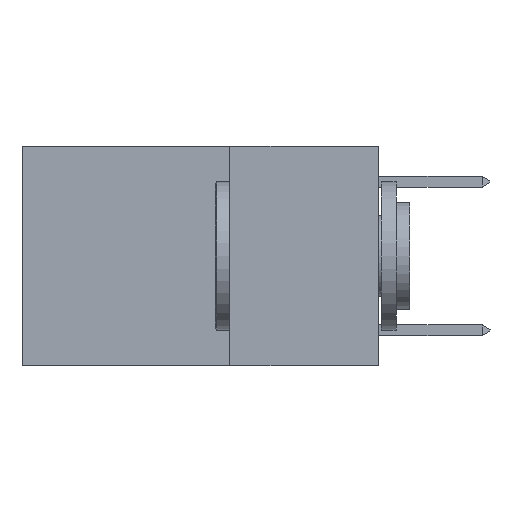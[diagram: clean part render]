
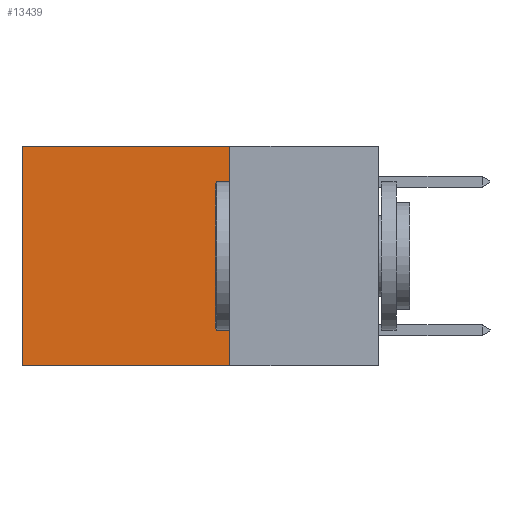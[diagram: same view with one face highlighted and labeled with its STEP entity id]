
A CAD part, left-side view. The second image highlights one B-rep face of the part: STEP entity #13439.
In plain terms, the highlighted planar face has unit normal (-1, 0, 0).
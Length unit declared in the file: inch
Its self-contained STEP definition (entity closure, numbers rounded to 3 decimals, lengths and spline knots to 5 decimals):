
#74 = AXIS2_PLACEMENT_3D ( 'NONE', #9755, #10121, #9610 ) ;
#887 = CARTESIAN_POINT ( 'NONE',  ( 0.2625, 0.25, -0.37 ) ) ;
#1999 = VERTEX_POINT ( 'NONE', #17537 ) ;
#2059 = DIRECTION ( 'NONE',  ( 0., 1., 0. ) ) ;
#2319 = CARTESIAN_POINT ( 'NONE',  ( 0.2625, 0.25, -0.37 ) ) ;
#3209 = DIRECTION ( 'NONE',  ( 0., 0., -1. ) ) ;
#3644 = CARTESIAN_POINT ( 'NONE',  ( 0.2625, 0.25, 0. ) ) ;
#4474 = ORIENTED_EDGE ( 'NONE', *, *, #15202, .T. ) ;
#4477 = EDGE_LOOP ( 'NONE', ( #7351, #19749, #8187, #4474 ) ) ;
#4479 = DIRECTION ( 'NONE',  ( 0., 1., 0. ) ) ;
#4602 = CARTESIAN_POINT ( 'NONE',  ( 0.2625, 0.25, 0. ) ) ;
#4672 = CARTESIAN_POINT ( 'NONE',  ( 0.2625, 0.6, -0.37 ) ) ;
#5566 = VERTEX_POINT ( 'NONE', #7783 ) ;
#7351 = ORIENTED_EDGE ( 'NONE', *, *, #16400, .T. ) ;
#7783 = CARTESIAN_POINT ( 'NONE',  ( 0.2625, 0.6, 0. ) ) ;
#8187 = ORIENTED_EDGE ( 'NONE', *, *, #9574, .F. ) ;
#8329 = VECTOR ( 'NONE', #17251, 39.37008 ) ;
#8354 = LINE ( 'NONE', #16180, #8329 ) ;
#8377 = FACE_OUTER_BOUND ( 'NONE', #4477, .T. ) ;
#9574 = EDGE_CURVE ( 'NONE', #1999, #19134, #17274, .T. ) ;
#9610 = DIRECTION ( 'NONE',  ( 0., 0., -1. ) ) ;
#9755 = CARTESIAN_POINT ( 'NONE',  ( 0.2625, 0.25, 0. ) ) ;
#10121 = DIRECTION ( 'NONE',  ( 1., 0., 0. ) ) ;
#10165 = VECTOR ( 'NONE', #2059, 39.37008 ) ;
#10316 = LINE ( 'NONE', #2319, #10165 ) ;
#10623 = EDGE_CURVE ( 'NONE', #19134, #13665, #10316, .T. ) ;
#11141 = PLANE ( 'NONE',  #74 ) ;
#13439 = ADVANCED_FACE ( 'NONE', ( #8377 ), #11141, .F. ) ;
#13665 = VERTEX_POINT ( 'NONE', #4672 ) ;
#15202 = EDGE_CURVE ( 'NONE', #1999, #5566, #15602, .T. ) ;
#15489 = VECTOR ( 'NONE', #4479, 39.37008 ) ;
#15602 = LINE ( 'NONE', #4602, #15489 ) ;
#16180 = CARTESIAN_POINT ( 'NONE',  ( 0.2625, 0.6, 0. ) ) ;
#16400 = EDGE_CURVE ( 'NONE', #5566, #13665, #8354, .T. ) ;
#17201 = VECTOR ( 'NONE', #3209, 39.37008 ) ;
#17251 = DIRECTION ( 'NONE',  ( 0., 0., -1. ) ) ;
#17274 = LINE ( 'NONE', #3644, #17201 ) ;
#17537 = CARTESIAN_POINT ( 'NONE',  ( 0.2625, 0.25, 0. ) ) ;
#19134 = VERTEX_POINT ( 'NONE', #887 ) ;
#19749 = ORIENTED_EDGE ( 'NONE', *, *, #10623, .F. ) ;
